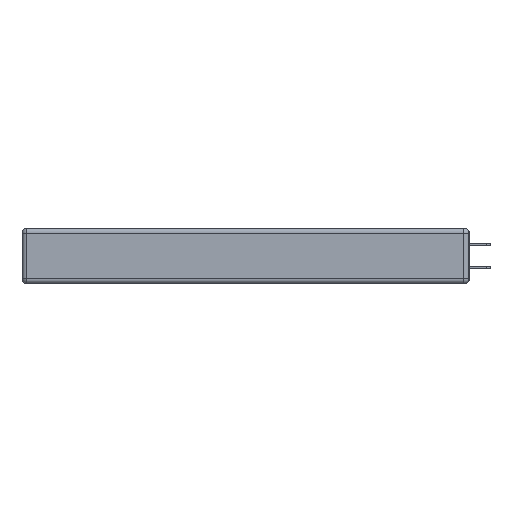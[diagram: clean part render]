
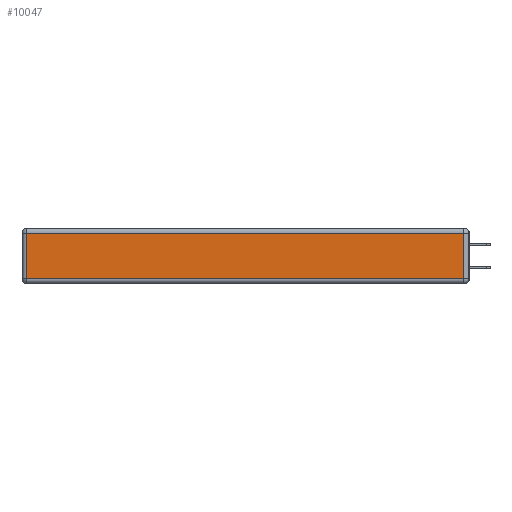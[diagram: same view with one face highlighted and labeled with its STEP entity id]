
A CAD part, left-side view. The second image highlights one B-rep face of the part: STEP entity #10047.
In plain terms, the highlighted planar face has unit normal (-1, 0, 0).
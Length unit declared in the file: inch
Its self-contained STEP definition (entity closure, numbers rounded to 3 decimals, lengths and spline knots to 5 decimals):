
#1025 = ORIENTED_EDGE ( 'NONE', *, *, #5176, .T. ) ;
#2354 = VERTEX_POINT ( 'NONE', #15131 ) ;
#2871 = CARTESIAN_POINT ( 'NONE',  ( 0., 2.75, -0.03 ) ) ;
#3495 = CARTESIAN_POINT ( 'NONE',  ( 0., 2.72, -0.03 ) ) ;
#3829 = DIRECTION ( 'NONE',  ( 0., -1., 0. ) ) ;
#3986 = LINE ( 'NONE', #4335, #7380 ) ;
#4047 = CARTESIAN_POINT ( 'NONE',  ( 0., 0., -0.313 ) ) ;
#4335 = CARTESIAN_POINT ( 'NONE',  ( 0., 0.03, -0.343 ) ) ;
#5176 = EDGE_CURVE ( 'NONE', #2354, #21736, #9097, .T. ) ;
#5327 = DIRECTION ( 'NONE',  ( 0., 0., -1. ) ) ;
#6102 = EDGE_CURVE ( 'NONE', #21736, #14273, #3986, .T. ) ;
#6708 = VECTOR ( 'NONE', #5327, 39.37008 ) ;
#7380 = VECTOR ( 'NONE', #9809, 39.37008 ) ;
#7647 = ORIENTED_EDGE ( 'NONE', *, *, #8349, .T. ) ;
#8349 = EDGE_CURVE ( 'NONE', #14273, #18444, #20437, .T. ) ;
#8713 = VECTOR ( 'NONE', #10673, 39.37008 ) ;
#9097 = LINE ( 'NONE', #4047, #16357 ) ;
#9782 = FACE_OUTER_BOUND ( 'NONE', #13838, .T. ) ;
#9809 = DIRECTION ( 'NONE',  ( 0., 0., 1. ) ) ;
#9867 = ORIENTED_EDGE ( 'NONE', *, *, #10139, .T. ) ;
#10047 = ADVANCED_FACE ( 'NONE', ( #9782 ), #11411, .T. ) ;
#10139 = EDGE_CURVE ( 'NONE', #18444, #2354, #14509, .T. ) ;
#10396 = CARTESIAN_POINT ( 'NONE',  ( 0., 2.72, -0.343 ) ) ;
#10673 = DIRECTION ( 'NONE',  ( 0., 1., 0. ) ) ;
#10826 = AXIS2_PLACEMENT_3D ( 'NONE', #11333, #16918, #18635 ) ;
#11333 = CARTESIAN_POINT ( 'NONE',  ( 0., 0., -0.343 ) ) ;
#11411 = PLANE ( 'NONE',  #10826 ) ;
#13838 = EDGE_LOOP ( 'NONE', ( #1025, #20356, #7647, #9867 ) ) ;
#14273 = VERTEX_POINT ( 'NONE', #17568 ) ;
#14509 = LINE ( 'NONE', #10396, #6708 ) ;
#15131 = CARTESIAN_POINT ( 'NONE',  ( 0., 2.72, -0.313 ) ) ;
#16357 = VECTOR ( 'NONE', #3829, 39.37008 ) ;
#16918 = DIRECTION ( 'NONE',  ( -1., 0., 0. ) ) ;
#17568 = CARTESIAN_POINT ( 'NONE',  ( 0., 0.03, -0.03 ) ) ;
#18444 = VERTEX_POINT ( 'NONE', #3495 ) ;
#18635 = DIRECTION ( 'NONE',  ( 0., 0., 1. ) ) ;
#18880 = CARTESIAN_POINT ( 'NONE',  ( 0., 0.03, -0.313 ) ) ;
#20356 = ORIENTED_EDGE ( 'NONE', *, *, #6102, .T. ) ;
#20437 = LINE ( 'NONE', #2871, #8713 ) ;
#21736 = VERTEX_POINT ( 'NONE', #18880 ) ;
